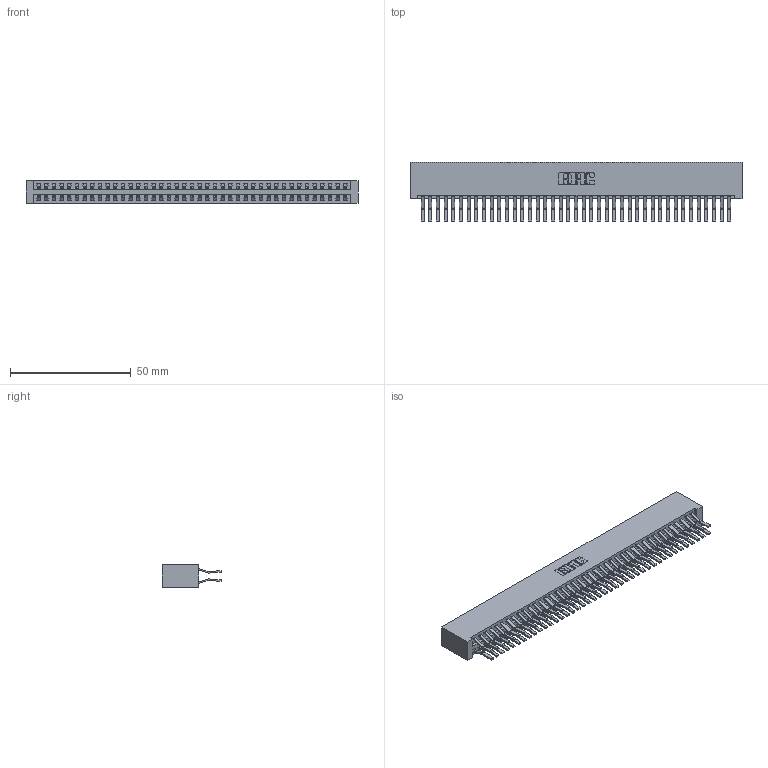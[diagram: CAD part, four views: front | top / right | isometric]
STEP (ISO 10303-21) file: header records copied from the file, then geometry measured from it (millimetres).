
FILE_DESCRIPTION (( 'STEP AP203' ), '1' );
FILE_NAME ('346-082-560-201.STEP', '2022-05-25T18:53:03', ( '' ), ( '' ), 'SwSTEP 2.0', 'SolidWorks 2020', '' );
FILE_SCHEMA (( 'CONFIG_CONTROL_DESIGN' ));
Length unit declared in the file: inch
Products named in the file (3): 346-082-560-201; 345-292-001_560 Tail; 346 Part_No Mounting Lugs
Assembly tree (83 placements, depth 2):
  346-082-560-201
    346 Part_No Mounting Lugs
    345-292-001_560 Tail  x82
Bounding box: 137.41 x 24.78 x 9.4 mm (x, y, z)
Volume: 14502.6 mm3; surface area: 21516.2 mm2
Topology: 83 solids, 83 shells, 4542 faces, 13507 edges, 8894 vertices
Faces by surface type: plane 2942, cylinder 1600
Entity records: 26703 total; most frequent: CARTESIAN_POINT 4400, ORIENTED_EDGE 4334, DIRECTION 3927, EDGE_CURVE 2167, VECTOR 1875, LINE 1875, VERTEX_POINT 1442, AXIS2_PLACEMENT_3D 1026
